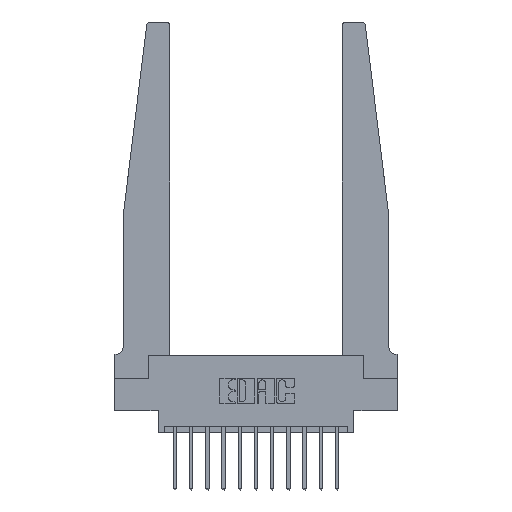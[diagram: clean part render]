
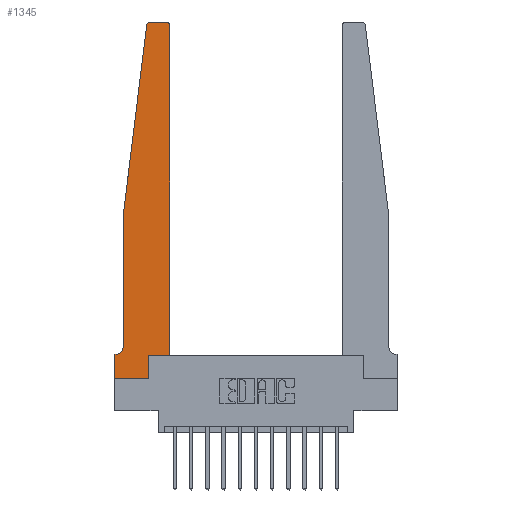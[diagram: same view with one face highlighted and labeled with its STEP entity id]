
A CAD part, top view. The second image highlights one B-rep face of the part: STEP entity #1345.
In plain terms, the highlighted planar face has unit normal (0, 0, 1).
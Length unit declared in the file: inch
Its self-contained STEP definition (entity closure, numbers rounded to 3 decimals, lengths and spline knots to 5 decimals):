
#3 = AXIS2_PLACEMENT_3D ( 'NONE', #6026, #9965, #9787 ) ;
#20 = ORIENTED_EDGE ( 'NONE', *, *, #6873, .T. ) ;
#281 = EDGE_CURVE ( 'NONE', #742, #2158, #5372, .T. ) ;
#478 = CARTESIAN_POINT ( 'NONE',  ( 0.065, 0.1875, 0.37 ) ) ;
#704 = CARTESIAN_POINT ( 'NONE',  ( 0., 0., 0.37 ) ) ;
#742 = VERTEX_POINT ( 'NONE', #13340 ) ;
#956 = CARTESIAN_POINT ( 'NONE',  ( 0.015, 0.2375, 0.37 ) ) ;
#1167 = DIRECTION ( 'NONE',  ( 1., 0., 0. ) ) ;
#1345 = ADVANCED_FACE ( 'NONE', ( #9119 ), #15378, .T. ) ;
#1802 = CARTESIAN_POINT ( 'NONE',  ( 0.065, 1.25, 0.37 ) ) ;
#2072 = CARTESIAN_POINT ( 'NONE',  ( 0.425, 0.18, 0.37 ) ) ;
#2158 = VERTEX_POINT ( 'NONE', #9086 ) ;
#2214 = VECTOR ( 'NONE', #9569, 39.37008 ) ;
#2338 = VERTEX_POINT ( 'NONE', #15476 ) ;
#2410 = CARTESIAN_POINT ( 'NONE',  ( 0., 0., 0.37 ) ) ;
#2528 = AXIS2_PLACEMENT_3D ( 'NONE', #956, #3686, #6252 ) ;
#3079 = VERTEX_POINT ( 'NONE', #6807 ) ;
#3686 = DIRECTION ( 'NONE',  ( 0., 0., -1. ) ) ;
#3708 = VERTEX_POINT ( 'NONE', #14925 ) ;
#3755 = DIRECTION ( 'NONE',  ( 0., -1., 0. ) ) ;
#3843 = CARTESIAN_POINT ( 'NONE',  ( 0., 0.1875, 0.37 ) ) ;
#4017 = VERTEX_POINT ( 'NONE', #4317 ) ;
#4077 = EDGE_CURVE ( 'NONE', #7243, #11783, #14585, .T. ) ;
#4253 = LINE ( 'NONE', #5591, #7318 ) ;
#4317 = CARTESIAN_POINT ( 'NONE',  ( 0.2605, 0., 0.37 ) ) ;
#4469 = CARTESIAN_POINT ( 'NONE',  ( 0.2605, 0.18, 0.37 ) ) ;
#4519 = CARTESIAN_POINT ( 'NONE',  ( 0.015, 0.1875, 0.37 ) ) ;
#4844 = LINE ( 'NONE', #6091, #8393 ) ;
#5048 = ORIENTED_EDGE ( 'NONE', *, *, #11936, .T. ) ;
#5214 = VERTEX_POINT ( 'NONE', #12122 ) ;
#5227 = ORIENTED_EDGE ( 'NONE', *, *, #7873, .T. ) ;
#5372 = LINE ( 'NONE', #1802, #11096 ) ;
#5433 = VECTOR ( 'NONE', #5646, 39.37008 ) ;
#5591 = CARTESIAN_POINT ( 'NONE',  ( 0.065, 1.25, 0.37 ) ) ;
#5646 = DIRECTION ( 'NONE',  ( -1., 0., 0. ) ) ;
#5683 = CIRCLE ( 'NONE', #3, 0.03 ) ;
#5878 = CARTESIAN_POINT ( 'NONE',  ( 0.425, 2.72, 0.37 ) ) ;
#6026 = CARTESIAN_POINT ( 'NONE',  ( 0.395, 2.72, 0.37 ) ) ;
#6091 = CARTESIAN_POINT ( 'NONE',  ( 0.25, 2.75, 0.37 ) ) ;
#6113 = DIRECTION ( 'NONE',  ( 0., 1., 0. ) ) ;
#6252 = DIRECTION ( 'NONE',  ( -1., 0., 0. ) ) ;
#6325 = EDGE_CURVE ( 'NONE', #15985, #3708, #5683, .T. ) ;
#6374 = VERTEX_POINT ( 'NONE', #8544 ) ;
#6807 = CARTESIAN_POINT ( 'NONE',  ( 0.065, 0.2375, 0.37 ) ) ;
#6873 = EDGE_CURVE ( 'NONE', #11716, #2338, #13035, .T. ) ;
#6974 = VECTOR ( 'NONE', #3755, 39.37008 ) ;
#7018 = DIRECTION ( 'NONE',  ( -0.122, -0.992, 0. ) ) ;
#7243 = VERTEX_POINT ( 'NONE', #16132 ) ;
#7318 = VECTOR ( 'NONE', #11694, 39.37008 ) ;
#7441 = EDGE_CURVE ( 'NONE', #4017, #7243, #10837, .T. ) ;
#7530 = EDGE_CURVE ( 'NONE', #11783, #15985, #10992, .T. ) ;
#7873 = EDGE_CURVE ( 'NONE', #3708, #6374, #4844, .T. ) ;
#8021 = EDGE_LOOP ( 'NONE', ( #5227, #10705, #14059, #12056, #5048, #20, #16263, #15163, #15641, #12717, #11339, #16527 ) ) ;
#8197 = DIRECTION ( 'NONE',  ( 1., 0., 0. ) ) ;
#8201 = EDGE_CURVE ( 'NONE', #2158, #3079, #4253, .T. ) ;
#8280 = DIRECTION ( 'NONE',  ( -1., 0., 0. ) ) ;
#8393 = VECTOR ( 'NONE', #8280, 39.37008 ) ;
#8544 = CARTESIAN_POINT ( 'NONE',  ( 0.27653, 2.75, 0.37 ) ) ;
#8548 = LINE ( 'NONE', #704, #9523 ) ;
#8667 = AXIS2_PLACEMENT_3D ( 'NONE', #8921, #12794, #1167 ) ;
#8921 = CARTESIAN_POINT ( 'NONE',  ( 0.27653, 2.72, 0.37 ) ) ;
#9086 = CARTESIAN_POINT ( 'NONE',  ( 0.065, 1.25, 0.37 ) ) ;
#9119 = FACE_OUTER_BOUND ( 'NONE', #8021, .T. ) ;
#9489 = EDGE_CURVE ( 'NONE', #6374, #742, #15934, .T. ) ;
#9523 = VECTOR ( 'NONE', #11068, 39.37008 ) ;
#9533 = CARTESIAN_POINT ( 'NONE',  ( 0.425, 0.18, 0.37 ) ) ;
#9569 = DIRECTION ( 'NONE',  ( 0., 1., 0. ) ) ;
#9754 = CIRCLE ( 'NONE', #2528, 0.05 ) ;
#9787 = DIRECTION ( 'NONE',  ( 1., 0., 0. ) ) ;
#9848 = AXIS2_PLACEMENT_3D ( 'NONE', #3843, #14238, #12905 ) ;
#9965 = DIRECTION ( 'NONE',  ( 0., 0., 1. ) ) ;
#10281 = VECTOR ( 'NONE', #8197, 39.37008 ) ;
#10705 = ORIENTED_EDGE ( 'NONE', *, *, #9489, .T. ) ;
#10837 = LINE ( 'NONE', #4469, #2214 ) ;
#10992 = LINE ( 'NONE', #2072, #11338 ) ;
#11068 = DIRECTION ( 'NONE',  ( 1., 0., 0. ) ) ;
#11096 = VECTOR ( 'NONE', #7018, 39.37008 ) ;
#11338 = VECTOR ( 'NONE', #6113, 39.37008 ) ;
#11339 = ORIENTED_EDGE ( 'NONE', *, *, #7530, .T. ) ;
#11694 = DIRECTION ( 'NONE',  ( 0., -1., 0. ) ) ;
#11716 = VERTEX_POINT ( 'NONE', #4519 ) ;
#11783 = VERTEX_POINT ( 'NONE', #14775 ) ;
#11936 = EDGE_CURVE ( 'NONE', #3079, #11716, #9754, .T. ) ;
#11999 = EDGE_CURVE ( 'NONE', #2338, #5214, #15202, .T. ) ;
#12056 = ORIENTED_EDGE ( 'NONE', *, *, #8201, .T. ) ;
#12122 = CARTESIAN_POINT ( 'NONE',  ( 0., 0., 0.37 ) ) ;
#12717 = ORIENTED_EDGE ( 'NONE', *, *, #4077, .T. ) ;
#12794 = DIRECTION ( 'NONE',  ( 0., 0., 1. ) ) ;
#12905 = DIRECTION ( 'NONE',  ( 1., 0., 0. ) ) ;
#12940 = EDGE_CURVE ( 'NONE', #5214, #4017, #8548, .T. ) ;
#13035 = LINE ( 'NONE', #478, #5433 ) ;
#13340 = CARTESIAN_POINT ( 'NONE',  ( 0.24675, 2.72367, 0.37 ) ) ;
#14059 = ORIENTED_EDGE ( 'NONE', *, *, #281, .T. ) ;
#14238 = DIRECTION ( 'NONE',  ( 0., 0., 1. ) ) ;
#14585 = LINE ( 'NONE', #9533, #10281 ) ;
#14775 = CARTESIAN_POINT ( 'NONE',  ( 0.425, 0.18, 0.37 ) ) ;
#14925 = CARTESIAN_POINT ( 'NONE',  ( 0.395, 2.75, 0.37 ) ) ;
#15163 = ORIENTED_EDGE ( 'NONE', *, *, #12940, .T. ) ;
#15202 = LINE ( 'NONE', #2410, #6974 ) ;
#15378 = PLANE ( 'NONE',  #9848 ) ;
#15476 = CARTESIAN_POINT ( 'NONE',  ( 0., 0.1875, 0.37 ) ) ;
#15641 = ORIENTED_EDGE ( 'NONE', *, *, #7441, .T. ) ;
#15934 = CIRCLE ( 'NONE', #8667, 0.03 ) ;
#15985 = VERTEX_POINT ( 'NONE', #5878 ) ;
#16132 = CARTESIAN_POINT ( 'NONE',  ( 0.2605, 0.18, 0.37 ) ) ;
#16263 = ORIENTED_EDGE ( 'NONE', *, *, #11999, .T. ) ;
#16527 = ORIENTED_EDGE ( 'NONE', *, *, #6325, .T. ) ;
